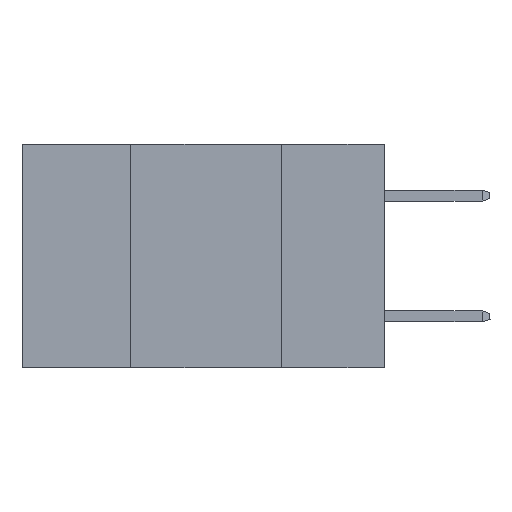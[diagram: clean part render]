
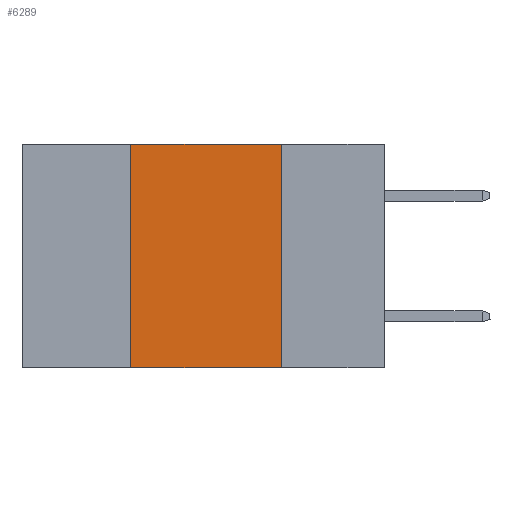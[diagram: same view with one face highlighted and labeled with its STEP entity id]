
A CAD part, left-side view. The second image highlights one B-rep face of the part: STEP entity #6289.
In plain terms, the highlighted planar face has unit normal (-1, 0, 0).
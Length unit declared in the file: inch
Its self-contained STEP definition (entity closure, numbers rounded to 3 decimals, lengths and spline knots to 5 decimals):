
#310 = VERTEX_POINT ( 'NONE', #23580 ) ;
#349 = ORIENTED_EDGE ( 'NONE', *, *, #22124, .F. ) ;
#1062 = PLANE ( 'NONE',  #8064 ) ;
#3436 = EDGE_CURVE ( 'NONE', #20274, #20410, #9085, .T. ) ;
#3984 = CARTESIAN_POINT ( 'NONE',  ( 0., 0.42, -0.37 ) ) ;
#4331 = VECTOR ( 'NONE', #13338, 39.37008 ) ;
#6289 = ADVANCED_FACE ( 'NONE', ( #21063 ), #1062, .F. ) ;
#7636 = CARTESIAN_POINT ( 'NONE',  ( 0., 0.17, 0. ) ) ;
#7922 = DIRECTION ( 'NONE',  ( 0., 0., -1. ) ) ;
#8064 = AXIS2_PLACEMENT_3D ( 'NONE', #8130, #28884, #7922 ) ;
#8130 = CARTESIAN_POINT ( 'NONE',  ( 0., 0.6, 0. ) ) ;
#9085 = LINE ( 'NONE', #11260, #4331 ) ;
#10141 = ORIENTED_EDGE ( 'NONE', *, *, #3436, .T. ) ;
#10150 = LINE ( 'NONE', #24725, #18522 ) ;
#10387 = CARTESIAN_POINT ( 'NONE',  ( 0., 0.17, -0.37 ) ) ;
#11260 = CARTESIAN_POINT ( 'NONE',  ( 0., 0.6, -0.37 ) ) ;
#11914 = EDGE_CURVE ( 'NONE', #310, #20410, #21097, .T. ) ;
#12118 = ORIENTED_EDGE ( 'NONE', *, *, #11914, .F. ) ;
#13338 = DIRECTION ( 'NONE',  ( 0., -1., 0. ) ) ;
#13683 = VECTOR ( 'NONE', #26247, 39.37008 ) ;
#14892 = EDGE_CURVE ( 'NONE', #20274, #17943, #28585, .T. ) ;
#14960 = VECTOR ( 'NONE', #21906, 39.37008 ) ;
#16511 = EDGE_LOOP ( 'NONE', ( #12118, #349, #29845, #10141 ) ) ;
#17665 = CARTESIAN_POINT ( 'NONE',  ( 0., 0.42, 0. ) ) ;
#17943 = VERTEX_POINT ( 'NONE', #24418 ) ;
#18522 = VECTOR ( 'NONE', #27752, 39.37008 ) ;
#20274 = VERTEX_POINT ( 'NONE', #3984 ) ;
#20410 = VERTEX_POINT ( 'NONE', #10387 ) ;
#21063 = FACE_OUTER_BOUND ( 'NONE', #16511, .T. ) ;
#21097 = LINE ( 'NONE', #7636, #14960 ) ;
#21906 = DIRECTION ( 'NONE',  ( 0., 0., -1. ) ) ;
#22124 = EDGE_CURVE ( 'NONE', #17943, #310, #10150, .T. ) ;
#23580 = CARTESIAN_POINT ( 'NONE',  ( 0., 0.17, 0. ) ) ;
#24418 = CARTESIAN_POINT ( 'NONE',  ( 0., 0.42, 0. ) ) ;
#24725 = CARTESIAN_POINT ( 'NONE',  ( 0., 0.6, 0. ) ) ;
#26247 = DIRECTION ( 'NONE',  ( 0., 0., 1. ) ) ;
#27752 = DIRECTION ( 'NONE',  ( 0., -1., 0. ) ) ;
#28585 = LINE ( 'NONE', #17665, #13683 ) ;
#28884 = DIRECTION ( 'NONE',  ( 1., 0., 0. ) ) ;
#29845 = ORIENTED_EDGE ( 'NONE', *, *, #14892, .F. ) ;
